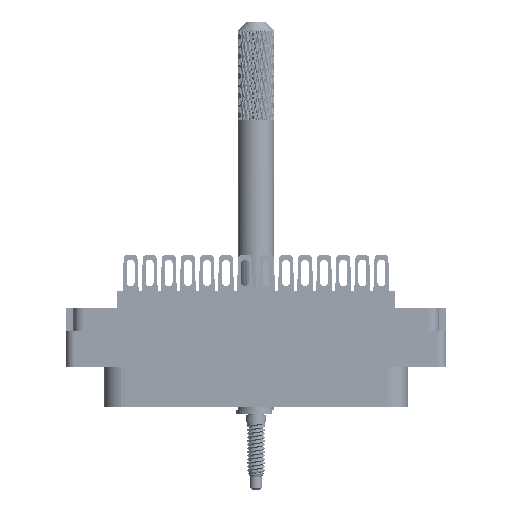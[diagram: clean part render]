
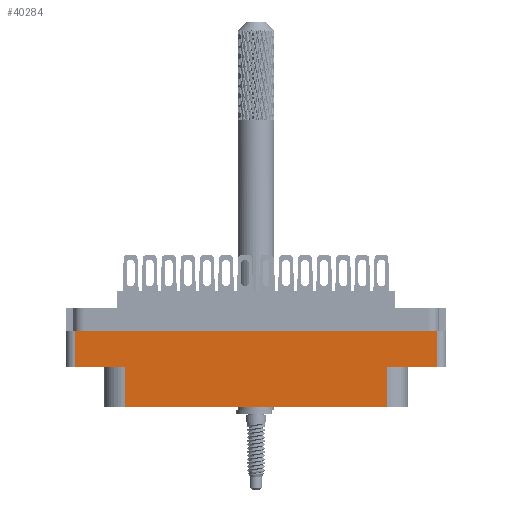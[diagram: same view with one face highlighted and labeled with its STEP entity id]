
A CAD part, front view. The second image highlights one B-rep face of the part: STEP entity #40284.
In plain terms, the highlighted planar face has unit normal (0, -1, 0).
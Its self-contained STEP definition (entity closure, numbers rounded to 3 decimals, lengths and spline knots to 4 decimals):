
#1088 = DIRECTION ( 'NONE',  ( -1., 0., 0. ) ) ;
#3156 = VECTOR ( 'NONE', #26371, 39.3701 ) ;
#4596 = VERTEX_POINT ( 'NONE', #108817 ) ;
#12741 = CARTESIAN_POINT ( 'NONE',  ( -1.2955, -0.438, -0.789 ) ) ;
#13031 = DIRECTION ( 'NONE',  ( 0., 0., -1. ) ) ;
#17178 = VERTEX_POINT ( 'NONE', #91228 ) ;
#18643 = CARTESIAN_POINT ( 'NONE',  ( 0., -0.438, -0.52 ) ) ;
#25177 = CARTESIAN_POINT ( 'NONE',  ( 0., -0.438, -0.52 ) ) ;
#26371 = DIRECTION ( 'NONE',  ( 0., 0., -1. ) ) ;
#27000 = DIRECTION ( 'NONE',  ( 0., 0., -1. ) ) ;
#27086 = CARTESIAN_POINT ( 'NONE',  ( 0.895, -0.438, -0.52 ) ) ;
#27446 = CARTESIAN_POINT ( 'NONE',  ( 0.895, -0.438, -0.52 ) ) ;
#27645 = EDGE_CURVE ( 'NONE', #4596, #50981, #50593, .T. ) ;
#28465 = CARTESIAN_POINT ( 'NONE',  ( 0.895, -0.438, -0.789 ) ) ;
#28912 = LINE ( 'NONE', #27446, #75015 ) ;
#29509 = DIRECTION ( 'NONE',  ( 1., 0., 0. ) ) ;
#30837 = AXIS2_PLACEMENT_3D ( 'NONE', #35935, #98655, #27000 ) ;
#35935 = CARTESIAN_POINT ( 'NONE',  ( -1.2955, -0.438, -0.789 ) ) ;
#35953 = ORIENTED_EDGE ( 'NONE', *, *, #60596, .T. ) ;
#37420 = FACE_OUTER_BOUND ( 'NONE', #78039, .T. ) ;
#37812 = VECTOR ( 'NONE', #29509, 39.3701 ) ;
#40250 = CARTESIAN_POINT ( 'NONE',  ( -0.895, -0.438, -0.789 ) ) ;
#40284 = ADVANCED_FACE ( 'NONE', ( #37420 ), #64010, .T. ) ;
#41564 = DIRECTION ( 'NONE',  ( 0., 0., 1. ) ) ;
#42805 = VECTOR ( 'NONE', #57566, 39.3701 ) ;
#42921 = VERTEX_POINT ( 'NONE', #65988 ) ;
#43844 = DIRECTION ( 'NONE',  ( -1., 0., 0. ) ) ;
#43904 = VECTOR ( 'NONE', #43844, 39.3701 ) ;
#44152 = CARTESIAN_POINT ( 'NONE',  ( -1.2335, -0.438, -0.52 ) ) ;
#45561 = LINE ( 'NONE', #75483, #42805 ) ;
#45746 = EDGE_CURVE ( 'NONE', #17178, #114368, #104797, .T. ) ;
#46488 = DIRECTION ( 'NONE',  ( 0., 0., 1. ) ) ;
#49843 = EDGE_CURVE ( 'NONE', #42921, #58127, #58333, .T. ) ;
#50593 = LINE ( 'NONE', #60707, #3156 ) ;
#50617 = ORIENTED_EDGE ( 'NONE', *, *, #66800, .F. ) ;
#50981 = VERTEX_POINT ( 'NONE', #44152 ) ;
#57566 = DIRECTION ( 'NONE',  ( 1., 0., 0. ) ) ;
#58127 = VERTEX_POINT ( 'NONE', #111842 ) ;
#58333 = LINE ( 'NONE', #84456, #94518 ) ;
#60596 = EDGE_CURVE ( 'NONE', #114368, #107003, #28912, .T. ) ;
#60707 = CARTESIAN_POINT ( 'NONE',  ( -1.2335, -0.438, -0.789 ) ) ;
#61601 = ORIENTED_EDGE ( 'NONE', *, *, #87111, .T. ) ;
#62924 = ORIENTED_EDGE ( 'NONE', *, *, #45746, .T. ) ;
#64010 = PLANE ( 'NONE',  #30837 ) ;
#65734 = VECTOR ( 'NONE', #13031, 39.3701 ) ;
#65988 = CARTESIAN_POINT ( 'NONE',  ( 1.2335, -0.438, -0.52 ) ) ;
#66800 = EDGE_CURVE ( 'NONE', #42921, #107003, #84381, .T. ) ;
#68906 = VERTEX_POINT ( 'NONE', #96623 ) ;
#75015 = VECTOR ( 'NONE', #46488, 39.3701 ) ;
#75483 = CARTESIAN_POINT ( 'NONE',  ( 0., -0.438, -0.274 ) ) ;
#78039 = EDGE_LOOP ( 'NONE', ( #100300, #86178, #90522, #61601, #62924, #35953, #50617, #79122 ) ) ;
#78858 = VECTOR ( 'NONE', #1088, 39.3701 ) ;
#79122 = ORIENTED_EDGE ( 'NONE', *, *, #49843, .T. ) ;
#84381 = LINE ( 'NONE', #18643, #78858 ) ;
#84456 = CARTESIAN_POINT ( 'NONE',  ( 1.2335, -0.438, -0.789 ) ) ;
#85277 = LINE ( 'NONE', #40250, #65734 ) ;
#86178 = ORIENTED_EDGE ( 'NONE', *, *, #27645, .T. ) ;
#87111 = EDGE_CURVE ( 'NONE', #68906, #17178, #85277, .T. ) ;
#90522 = ORIENTED_EDGE ( 'NONE', *, *, #106177, .F. ) ;
#91171 = EDGE_CURVE ( 'NONE', #4596, #58127, #45561, .T. ) ;
#91228 = CARTESIAN_POINT ( 'NONE',  ( -0.895, -0.438, -0.789 ) ) ;
#91285 = LINE ( 'NONE', #25177, #43904 ) ;
#94518 = VECTOR ( 'NONE', #41564, 39.3701 ) ;
#96623 = CARTESIAN_POINT ( 'NONE',  ( -0.895, -0.438, -0.52 ) ) ;
#98655 = DIRECTION ( 'NONE',  ( 0., -1., 0. ) ) ;
#100300 = ORIENTED_EDGE ( 'NONE', *, *, #91171, .F. ) ;
#104797 = LINE ( 'NONE', #12741, #37812 ) ;
#106177 = EDGE_CURVE ( 'NONE', #68906, #50981, #91285, .T. ) ;
#107003 = VERTEX_POINT ( 'NONE', #27086 ) ;
#108817 = CARTESIAN_POINT ( 'NONE',  ( -1.2335, -0.438, -0.274 ) ) ;
#111842 = CARTESIAN_POINT ( 'NONE',  ( 1.2335, -0.438, -0.274 ) ) ;
#114368 = VERTEX_POINT ( 'NONE', #28465 ) ;
